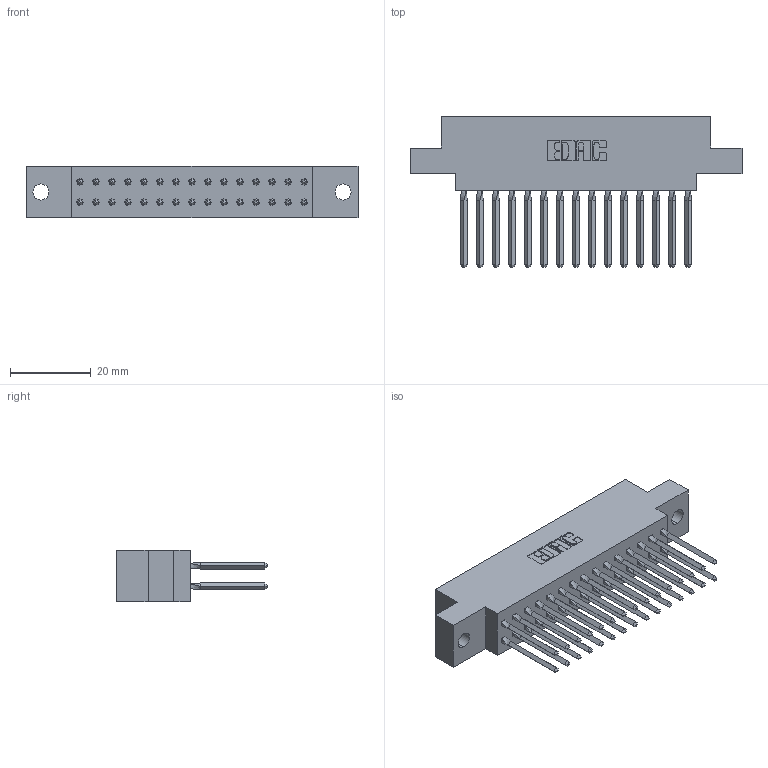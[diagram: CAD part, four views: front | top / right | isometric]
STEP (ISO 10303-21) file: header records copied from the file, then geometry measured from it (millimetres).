
FILE_DESCRIPTION (( 'STEP AP203' ), '1' );
FILE_NAME ('317-030-540-804.STEP', '2020-02-27T20:20:57', ( '' ), ( '' ), 'SwSTEP 2.0', 'SolidWorks 2016', '' );
FILE_SCHEMA (( 'CONFIG_CONTROL_DESIGN' ));
Length unit declared in the file: inch
Products named in the file (3): 317-290-001_540; 317-030-540-804; 317 Part_.156 Dia - TH
Assembly tree (31 placements, depth 2):
  317-030-540-804
    317 Part_.156 Dia - TH
    317-290-001_540  x30
Bounding box: 82.14 x 37.34 x 12.7 mm (x, y, z)
Volume: 12785.5 mm3; surface area: 17867.1 mm2
Topology: 31 solids, 31 shells, 2772 faces, 7685 edges, 4952 vertices
Faces by surface type: plane 2248, cylinder 404, bspline 120
Entity records: 25452 total; most frequent: CARTESIAN_POINT 4851, ORIENTED_EDGE 4350, DIRECTION 3633, EDGE_CURVE 2175, LINE 1919, VECTOR 1919, VERTEX_POINT 1443, AXIS2_PLACEMENT_3D 857
